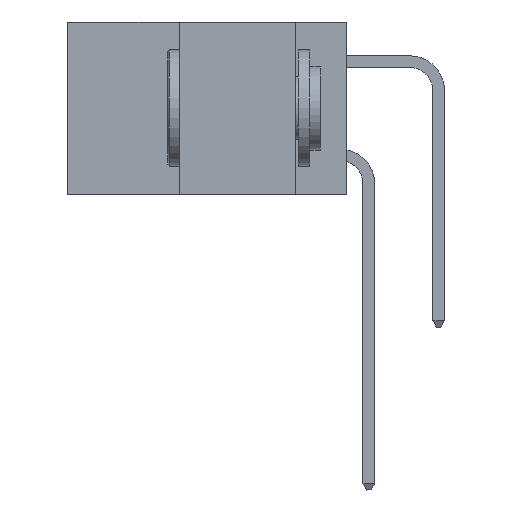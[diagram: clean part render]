
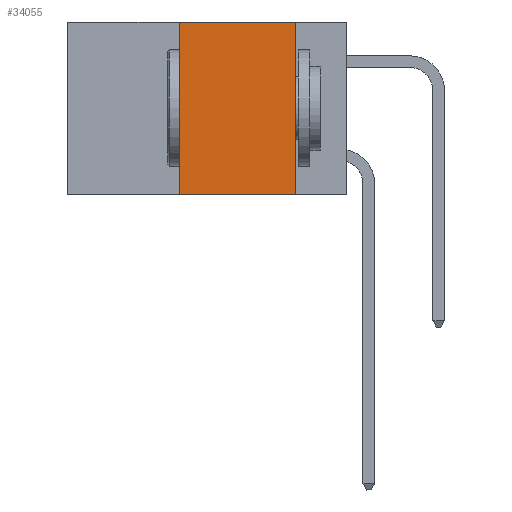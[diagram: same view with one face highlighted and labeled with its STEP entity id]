
A CAD part, left-side view. The second image highlights one B-rep face of the part: STEP entity #34055.
In plain terms, the highlighted planar face has unit normal (-1, 0, 0).
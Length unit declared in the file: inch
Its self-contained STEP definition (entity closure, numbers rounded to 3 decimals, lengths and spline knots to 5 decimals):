
#78 = CARTESIAN_POINT ( 'NONE',  ( 0., 0.6, -0.37 ) ) ;
#2807 = CARTESIAN_POINT ( 'NONE',  ( 0., 0.6, 0. ) ) ;
#3165 = FACE_OUTER_BOUND ( 'NONE', #14408, .T. ) ;
#3272 = ORIENTED_EDGE ( 'NONE', *, *, #28169, .F. ) ;
#4300 = LINE ( 'NONE', #29415, #13704 ) ;
#4707 = CARTESIAN_POINT ( 'NONE',  ( 0., 0.36, 0. ) ) ;
#4724 = DIRECTION ( 'NONE',  ( 0., -1., 0. ) ) ;
#5241 = VERTEX_POINT ( 'NONE', #23852 ) ;
#7631 = VERTEX_POINT ( 'NONE', #43759 ) ;
#8277 = DIRECTION ( 'NONE',  ( 0., 0., 1. ) ) ;
#10175 = ORIENTED_EDGE ( 'NONE', *, *, #39913, .F. ) ;
#10409 = CARTESIAN_POINT ( 'NONE',  ( 0., 0.36, -0.37 ) ) ;
#12331 = LINE ( 'NONE', #37953, #32154 ) ;
#13031 = VECTOR ( 'NONE', #8277, 39.37008 ) ;
#13318 = PLANE ( 'NONE',  #22210 ) ;
#13479 = DIRECTION ( 'NONE',  ( 0., 0., -1. ) ) ;
#13704 = VECTOR ( 'NONE', #4724, 39.37008 ) ;
#14408 = EDGE_LOOP ( 'NONE', ( #3272, #42642, #10175, #41055 ) ) ;
#15820 = CARTESIAN_POINT ( 'NONE',  ( 0., 0.11, 0. ) ) ;
#18658 = EDGE_CURVE ( 'NONE', #5241, #20621, #4300, .T. ) ;
#19000 = EDGE_CURVE ( 'NONE', #34148, #7631, #36162, .T. ) ;
#20621 = VERTEX_POINT ( 'NONE', #15820 ) ;
#22210 = AXIS2_PLACEMENT_3D ( 'NONE', #2807, #34456, #13479 ) ;
#23852 = CARTESIAN_POINT ( 'NONE',  ( 0., 0.36, 0. ) ) ;
#28169 = EDGE_CURVE ( 'NONE', #20621, #7631, #12331, .T. ) ;
#28336 = DIRECTION ( 'NONE',  ( 0., -1., 0. ) ) ;
#29415 = CARTESIAN_POINT ( 'NONE',  ( 0., 0.6, 0. ) ) ;
#30647 = LINE ( 'NONE', #4707, #13031 ) ;
#32154 = VECTOR ( 'NONE', #41367, 39.37008 ) ;
#32748 = VECTOR ( 'NONE', #28336, 39.37008 ) ;
#34055 = ADVANCED_FACE ( 'NONE', ( #3165 ), #13318, .F. ) ;
#34148 = VERTEX_POINT ( 'NONE', #10409 ) ;
#34456 = DIRECTION ( 'NONE',  ( 1., 0., 0. ) ) ;
#36162 = LINE ( 'NONE', #78, #32748 ) ;
#37953 = CARTESIAN_POINT ( 'NONE',  ( 0., 0.11, 0. ) ) ;
#39913 = EDGE_CURVE ( 'NONE', #34148, #5241, #30647, .T. ) ;
#41055 = ORIENTED_EDGE ( 'NONE', *, *, #19000, .T. ) ;
#41367 = DIRECTION ( 'NONE',  ( 0., 0., -1. ) ) ;
#42642 = ORIENTED_EDGE ( 'NONE', *, *, #18658, .F. ) ;
#43759 = CARTESIAN_POINT ( 'NONE',  ( 0., 0.11, -0.37 ) ) ;
